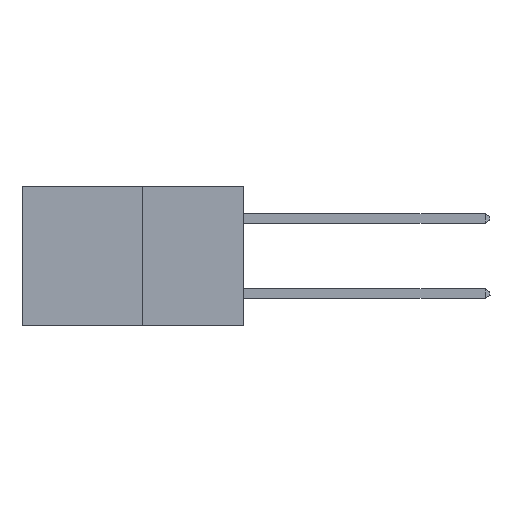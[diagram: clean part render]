
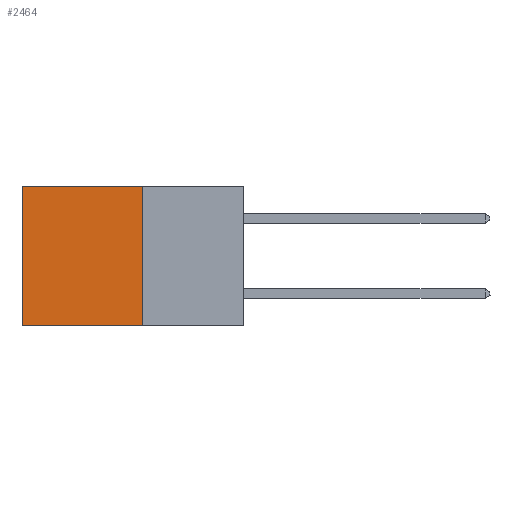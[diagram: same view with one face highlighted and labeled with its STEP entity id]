
A CAD part, left-side view. The second image highlights one B-rep face of the part: STEP entity #2464.
In plain terms, the highlighted planar face has unit normal (-1, 0, 0).
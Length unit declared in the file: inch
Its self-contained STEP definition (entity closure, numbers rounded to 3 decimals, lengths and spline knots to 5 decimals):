
#405 = VECTOR ( 'NONE', #4227, 39.37008 ) ;
#464 = EDGE_CURVE ( 'NONE', #6181, #19203, #10454, .T. ) ;
#1474 = AXIS2_PLACEMENT_3D ( 'NONE', #20731, #11306, #14992 ) ;
#2464 = ADVANCED_FACE ( 'NONE', ( #11670 ), #25418, .F. ) ;
#2546 = EDGE_CURVE ( 'NONE', #22905, #19203, #25331, .T. ) ;
#4227 = DIRECTION ( 'NONE',  ( 0., 0., -1. ) ) ;
#4809 = CARTESIAN_POINT ( 'NONE',  ( 0.277, 0.27, 0. ) ) ;
#5696 = CARTESIAN_POINT ( 'NONE',  ( 0.277, 0.59, 0. ) ) ;
#6181 = VERTEX_POINT ( 'NONE', #5696 ) ;
#8475 = VERTEX_POINT ( 'NONE', #19429 ) ;
#9076 = VECTOR ( 'NONE', #15101, 39.37008 ) ;
#10121 = CARTESIAN_POINT ( 'NONE',  ( 0.277, 0.27, -0.37 ) ) ;
#10454 = LINE ( 'NONE', #15541, #16493 ) ;
#11306 = DIRECTION ( 'NONE',  ( 1., 0., 0. ) ) ;
#11361 = LINE ( 'NONE', #12411, #405 ) ;
#11670 = FACE_OUTER_BOUND ( 'NONE', #16754, .T. ) ;
#11854 = LINE ( 'NONE', #4809, #21353 ) ;
#12411 = CARTESIAN_POINT ( 'NONE',  ( 0.277, 0.27, -0.37 ) ) ;
#13729 = ORIENTED_EDGE ( 'NONE', *, *, #464, .T. ) ;
#14733 = ORIENTED_EDGE ( 'NONE', *, *, #2546, .F. ) ;
#14992 = DIRECTION ( 'NONE',  ( 0., 0., -1. ) ) ;
#15077 = CARTESIAN_POINT ( 'NONE',  ( 0.277, 0.27, -0.37 ) ) ;
#15101 = DIRECTION ( 'NONE',  ( 0., 1., 0. ) ) ;
#15541 = CARTESIAN_POINT ( 'NONE',  ( 0.277, 0.59, -0.37 ) ) ;
#16493 = VECTOR ( 'NONE', #25890, 39.37008 ) ;
#16754 = EDGE_LOOP ( 'NONE', ( #13729, #14733, #26024, #24331 ) ) ;
#17195 = CARTESIAN_POINT ( 'NONE',  ( 0.277, 0.59, -0.37 ) ) ;
#17418 = EDGE_CURVE ( 'NONE', #8475, #22905, #11361, .T. ) ;
#19203 = VERTEX_POINT ( 'NONE', #17195 ) ;
#19429 = CARTESIAN_POINT ( 'NONE',  ( 0.277, 0.27, 0. ) ) ;
#20731 = CARTESIAN_POINT ( 'NONE',  ( 0.277, 0.27, -0.37 ) ) ;
#21353 = VECTOR ( 'NONE', #23084, 39.37008 ) ;
#22905 = VERTEX_POINT ( 'NONE', #10121 ) ;
#23084 = DIRECTION ( 'NONE',  ( 0., 1., 0. ) ) ;
#23202 = EDGE_CURVE ( 'NONE', #8475, #6181, #11854, .T. ) ;
#24331 = ORIENTED_EDGE ( 'NONE', *, *, #23202, .T. ) ;
#25331 = LINE ( 'NONE', #15077, #9076 ) ;
#25418 = PLANE ( 'NONE',  #1474 ) ;
#25890 = DIRECTION ( 'NONE',  ( 0., 0., -1. ) ) ;
#26024 = ORIENTED_EDGE ( 'NONE', *, *, #17418, .F. ) ;
